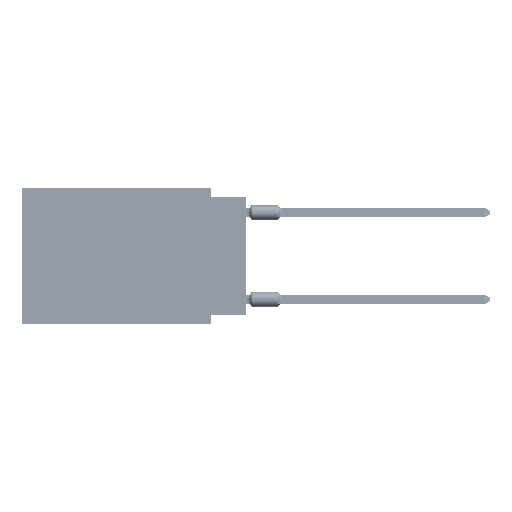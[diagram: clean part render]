
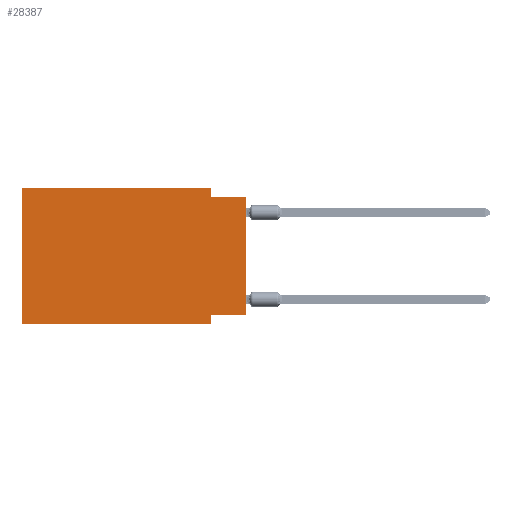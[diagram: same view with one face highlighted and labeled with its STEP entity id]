
A CAD part, left-side view. The second image highlights one B-rep face of the part: STEP entity #28387.
In plain terms, the highlighted planar face has unit normal (-1, 0, 0).
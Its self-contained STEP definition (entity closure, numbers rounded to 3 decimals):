
#2630 = DIRECTION ( 'NONE',  ( 0., 0., 1. ) ) ;
#3602 = DIRECTION ( 'NONE',  ( 0., 0., 1. ) ) ;
#3696 = DIRECTION ( 'NONE',  ( 0., -1., 0. ) ) ;
#4792 = VERTEX_POINT ( 'NONE', #8901 ) ;
#4941 = VECTOR ( 'NONE', #3696, 1000. ) ;
#5681 = EDGE_CURVE ( 'NONE', #6554, #4792, #34367, .T. ) ;
#5996 = EDGE_CURVE ( 'NONE', #17461, #28918, #17482, .T. ) ;
#6047 = CARTESIAN_POINT ( 'NONE',  ( 0., 0., -0.635 ) ) ;
#6554 = VERTEX_POINT ( 'NONE', #35514 ) ;
#7452 = EDGE_CURVE ( 'NONE', #6554, #12140, #9849, .T. ) ;
#8536 = EDGE_CURVE ( 'NONE', #52397, #28744, #29437, .T. ) ;
#8901 = CARTESIAN_POINT ( 'NONE',  ( 0., 16.383, 0. ) ) ;
#9849 = LINE ( 'NONE', #41297, #65381 ) ;
#10107 = EDGE_CURVE ( 'NONE', #36534, #12140, #52423, .T. ) ;
#10980 = VECTOR ( 'NONE', #68489, 1000. ) ;
#11705 = FACE_OUTER_BOUND ( 'NONE', #48286, .T. ) ;
#12140 = VERTEX_POINT ( 'NONE', #66959 ) ;
#12853 = ORIENTED_EDGE ( 'NONE', *, *, #5996, .F. ) ;
#17461 = VERTEX_POINT ( 'NONE', #45157 ) ;
#17482 = LINE ( 'NONE', #23072, #58587 ) ;
#17565 = ORIENTED_EDGE ( 'NONE', *, *, #8536, .T. ) ;
#20651 = VECTOR ( 'NONE', #2630, 1000. ) ;
#20975 = EDGE_CURVE ( 'NONE', #52397, #36534, #68730, .T. ) ;
#22467 = ORIENTED_EDGE ( 'NONE', *, *, #10107, .F. ) ;
#23072 = CARTESIAN_POINT ( 'NONE',  ( 0., 2.54, 0. ) ) ;
#27260 = ORIENTED_EDGE ( 'NONE', *, *, #49323, .F. ) ;
#28354 = CARTESIAN_POINT ( 'NONE',  ( 0., 2.54, -9.271 ) ) ;
#28387 = ADVANCED_FACE ( 'NONE', ( #11705 ), #54321, .F. ) ;
#28744 = VERTEX_POINT ( 'NONE', #6047 ) ;
#28918 = VERTEX_POINT ( 'NONE', #45840 ) ;
#29437 = LINE ( 'NONE', #29778, #58632 ) ;
#29778 = CARTESIAN_POINT ( 'NONE',  ( 0., 0., 0. ) ) ;
#30522 = CARTESIAN_POINT ( 'NONE',  ( 0., 16.383, 0. ) ) ;
#30994 = CARTESIAN_POINT ( 'NONE',  ( 0., 0., -9.271 ) ) ;
#31923 = DIRECTION ( 'NONE',  ( 0., -1., 0. ) ) ;
#32930 = LINE ( 'NONE', #54272, #61324 ) ;
#34367 = LINE ( 'NONE', #30522, #20651 ) ;
#34562 = DIRECTION ( 'NONE',  ( 0., 0., -1. ) ) ;
#35514 = CARTESIAN_POINT ( 'NONE',  ( 0., 16.383, -9.906 ) ) ;
#36534 = VERTEX_POINT ( 'NONE', #28354 ) ;
#38054 = EDGE_CURVE ( 'NONE', #28918, #28744, #50848, .T. ) ;
#41297 = CARTESIAN_POINT ( 'NONE',  ( 0., 16.383, -9.906 ) ) ;
#45157 = CARTESIAN_POINT ( 'NONE',  ( 0., 2.54, 0. ) ) ;
#45840 = CARTESIAN_POINT ( 'NONE',  ( 0., 2.54, -0.635 ) ) ;
#47101 = DIRECTION ( 'NONE',  ( 0., 1., 0. ) ) ;
#47911 = ORIENTED_EDGE ( 'NONE', *, *, #5681, .F. ) ;
#48286 = EDGE_LOOP ( 'NONE', ( #17565, #60452, #12853, #27260, #47911, #63388, #22467, #48685 ) ) ;
#48685 = ORIENTED_EDGE ( 'NONE', *, *, #20975, .F. ) ;
#49080 = CARTESIAN_POINT ( 'NONE',  ( 0., 16.383, 0. ) ) ;
#49323 = EDGE_CURVE ( 'NONE', #4792, #17461, #32930, .T. ) ;
#50472 = DIRECTION ( 'NONE',  ( 0., 0., -1. ) ) ;
#50848 = LINE ( 'NONE', #57143, #4941 ) ;
#52397 = VERTEX_POINT ( 'NONE', #67720 ) ;
#52423 = LINE ( 'NONE', #68143, #10980 ) ;
#54272 = CARTESIAN_POINT ( 'NONE',  ( 0., 16.383, 0. ) ) ;
#54321 = PLANE ( 'NONE',  #63240 ) ;
#57143 = CARTESIAN_POINT ( 'NONE',  ( 0., 0., -0.635 ) ) ;
#57370 = DIRECTION ( 'NONE',  ( 0., -1., 0. ) ) ;
#58587 = VECTOR ( 'NONE', #34562, 1000. ) ;
#58632 = VECTOR ( 'NONE', #3602, 1000. ) ;
#60452 = ORIENTED_EDGE ( 'NONE', *, *, #38054, .F. ) ;
#61324 = VECTOR ( 'NONE', #31923, 1000. ) ;
#63240 = AXIS2_PLACEMENT_3D ( 'NONE', #49080, #66871, #50472 ) ;
#63388 = ORIENTED_EDGE ( 'NONE', *, *, #7452, .T. ) ;
#65381 = VECTOR ( 'NONE', #57370, 1000. ) ;
#66041 = VECTOR ( 'NONE', #47101, 1000. ) ;
#66871 = DIRECTION ( 'NONE',  ( 1., 0., 0. ) ) ;
#66959 = CARTESIAN_POINT ( 'NONE',  ( 0., 2.54, -9.906 ) ) ;
#67720 = CARTESIAN_POINT ( 'NONE',  ( 0., 0., -9.271 ) ) ;
#68143 = CARTESIAN_POINT ( 'NONE',  ( 0., 2.54, -9.906 ) ) ;
#68489 = DIRECTION ( 'NONE',  ( 0., 0., -1. ) ) ;
#68730 = LINE ( 'NONE', #30994, #66041 ) ;
